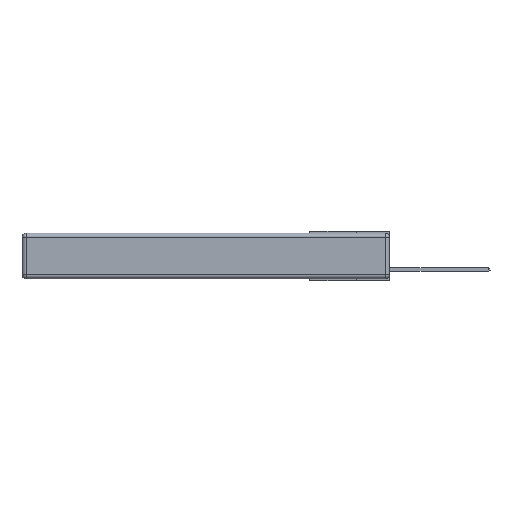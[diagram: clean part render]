
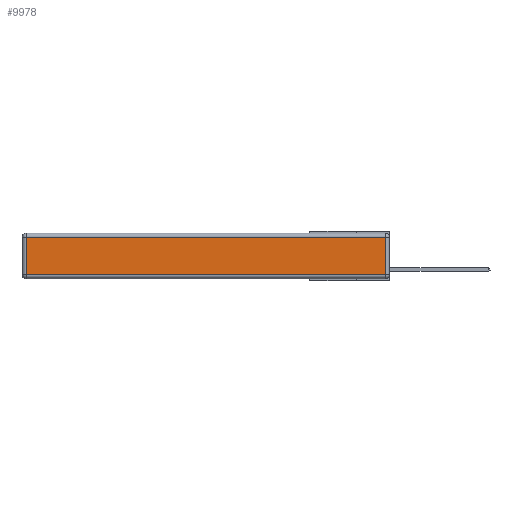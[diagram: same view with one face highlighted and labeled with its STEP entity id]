
A CAD part, left-side view. The second image highlights one B-rep face of the part: STEP entity #9978.
In plain terms, the highlighted planar face has unit normal (-1, 0, 0).
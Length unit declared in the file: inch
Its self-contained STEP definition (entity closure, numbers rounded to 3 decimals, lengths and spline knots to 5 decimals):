
#69 = EDGE_CURVE ( 'NONE', #12439, #12966, #9967, .T. ) ;
#456 = FACE_OUTER_BOUND ( 'NONE', #3310, .T. ) ;
#783 = CARTESIAN_POINT ( 'NONE',  ( 0., 0.03, -0.03 ) ) ;
#1140 = DIRECTION ( 'NONE',  ( -1., 0., 0. ) ) ;
#1950 = DIRECTION ( 'NONE',  ( 0., 0., 1. ) ) ;
#2004 = ORIENTED_EDGE ( 'NONE', *, *, #4478, .T. ) ;
#2742 = CARTESIAN_POINT ( 'NONE',  ( 0., 2.72, -0.343 ) ) ;
#3032 = LINE ( 'NONE', #9171, #8026 ) ;
#3116 = CARTESIAN_POINT ( 'NONE',  ( 0., 0., -0.313 ) ) ;
#3142 = VERTEX_POINT ( 'NONE', #8409 ) ;
#3184 = DIRECTION ( 'NONE',  ( 0., 0., 1. ) ) ;
#3306 = VECTOR ( 'NONE', #10576, 39.37008 ) ;
#3310 = EDGE_LOOP ( 'NONE', ( #10452, #6052, #4151, #2004 ) ) ;
#3749 = LINE ( 'NONE', #2742, #3909 ) ;
#3909 = VECTOR ( 'NONE', #7932, 39.37008 ) ;
#4151 = ORIENTED_EDGE ( 'NONE', *, *, #5761, .T. ) ;
#4478 = EDGE_CURVE ( 'NONE', #3142, #12439, #3749, .T. ) ;
#5325 = PLANE ( 'NONE',  #5425 ) ;
#5425 = AXIS2_PLACEMENT_3D ( 'NONE', #6367, #1140, #3184 ) ;
#5761 = EDGE_CURVE ( 'NONE', #13486, #3142, #3032, .T. ) ;
#6052 = ORIENTED_EDGE ( 'NONE', *, *, #10985, .T. ) ;
#6367 = CARTESIAN_POINT ( 'NONE',  ( 0., 0., -0.343 ) ) ;
#6404 = CARTESIAN_POINT ( 'NONE',  ( 0., 0.03, -0.343 ) ) ;
#7932 = DIRECTION ( 'NONE',  ( 0., 0., -1. ) ) ;
#8026 = VECTOR ( 'NONE', #12402, 39.37008 ) ;
#8272 = CARTESIAN_POINT ( 'NONE',  ( 0., 2.72, -0.313 ) ) ;
#8409 = CARTESIAN_POINT ( 'NONE',  ( 0., 2.72, -0.03 ) ) ;
#9171 = CARTESIAN_POINT ( 'NONE',  ( 0., 2.75, -0.03 ) ) ;
#9967 = LINE ( 'NONE', #3116, #3306 ) ;
#9978 = ADVANCED_FACE ( 'NONE', ( #456 ), #5325, .T. ) ;
#10404 = LINE ( 'NONE', #6404, #12243 ) ;
#10452 = ORIENTED_EDGE ( 'NONE', *, *, #69, .T. ) ;
#10576 = DIRECTION ( 'NONE',  ( 0., -1., 0. ) ) ;
#10985 = EDGE_CURVE ( 'NONE', #12966, #13486, #10404, .T. ) ;
#11150 = CARTESIAN_POINT ( 'NONE',  ( 0., 0.03, -0.313 ) ) ;
#12243 = VECTOR ( 'NONE', #1950, 39.37008 ) ;
#12402 = DIRECTION ( 'NONE',  ( 0., 1., 0. ) ) ;
#12439 = VERTEX_POINT ( 'NONE', #8272 ) ;
#12966 = VERTEX_POINT ( 'NONE', #11150 ) ;
#13486 = VERTEX_POINT ( 'NONE', #783 ) ;
